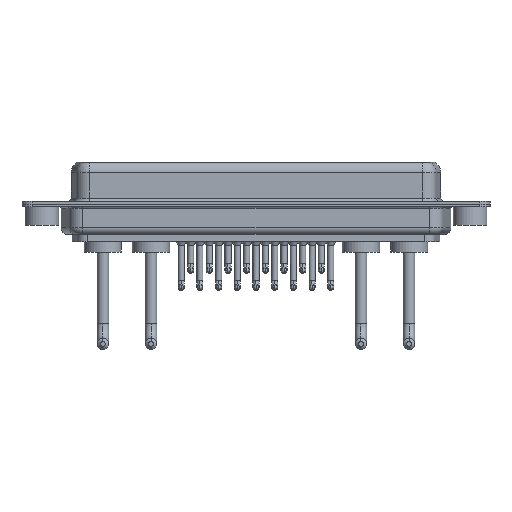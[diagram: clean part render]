
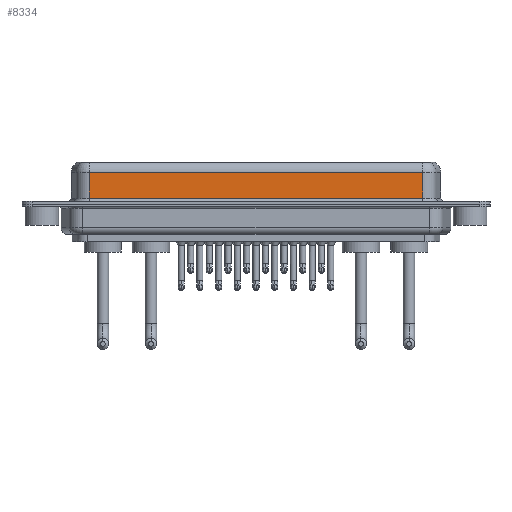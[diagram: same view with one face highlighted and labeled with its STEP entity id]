
A CAD part, front view. The second image highlights one B-rep face of the part: STEP entity #8334.
In plain terms, the highlighted planar face has unit normal (0, -1, 0).
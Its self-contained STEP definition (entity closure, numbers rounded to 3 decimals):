
#662 = ORIENTED_EDGE ( 'NONE', *, *, #8772, .T. ) ;
#1436 = DIRECTION ( 'NONE',  ( -1., 0., 0. ) ) ;
#1782 = DIRECTION ( 'NONE',  ( 0., 0., -1. ) ) ;
#2247 = ORIENTED_EDGE ( 'NONE', *, *, #20388, .F. ) ;
#2934 = EDGE_CURVE ( 'NONE', #20072, #3541, #20333, .T. ) ;
#3494 = CARTESIAN_POINT ( 'NONE',  ( 56.462, -3.95, 0.9 ) ) ;
#3541 = VERTEX_POINT ( 'NONE', #10389 ) ;
#3638 = ORIENTED_EDGE ( 'NONE', *, *, #15720, .T. ) ;
#3712 = PLANE ( 'NONE',  #6332 ) ;
#4052 = ORIENTED_EDGE ( 'NONE', *, *, #2934, .T. ) ;
#4742 = DIRECTION ( 'NONE',  ( 0., 0., 1. ) ) ;
#4967 = VERTEX_POINT ( 'NONE', #16690 ) ;
#5151 = LINE ( 'NONE', #8379, #12789 ) ;
#6005 = VECTOR ( 'NONE', #20217, 1000. ) ;
#6332 = AXIS2_PLACEMENT_3D ( 'NONE', #13130, #20021, #4742 ) ;
#6909 = CARTESIAN_POINT ( 'NONE',  ( 56.462, -3.95, 4.65 ) ) ;
#7437 = CARTESIAN_POINT ( 'NONE',  ( 7.038, -3.95, 4.65 ) ) ;
#7652 = CARTESIAN_POINT ( 'NONE',  ( 7.038, -3.95, 0.9 ) ) ;
#8334 = ADVANCED_FACE ( 'NONE', ( #14922 ), #3712, .F. ) ;
#8379 = CARTESIAN_POINT ( 'NONE',  ( 7.038, -3.95, 6.4 ) ) ;
#8772 = EDGE_CURVE ( 'NONE', #20502, #20072, #5151, .T. ) ;
#10389 = CARTESIAN_POINT ( 'NONE',  ( 56.462, -3.95, 0.9 ) ) ;
#11086 = CARTESIAN_POINT ( 'NONE',  ( 56.462, -3.95, 6.4 ) ) ;
#11422 = LINE ( 'NONE', #11086, #16417 ) ;
#12789 = VECTOR ( 'NONE', #1782, 1000. ) ;
#13130 = CARTESIAN_POINT ( 'NONE',  ( 56.462, -3.95, 6.4 ) ) ;
#14556 = DIRECTION ( 'NONE',  ( 0., 0., -1. ) ) ;
#14922 = FACE_OUTER_BOUND ( 'NONE', #15537, .T. ) ;
#15529 = VECTOR ( 'NONE', #1436, 1000. ) ;
#15537 = EDGE_LOOP ( 'NONE', ( #2247, #3638, #662, #4052 ) ) ;
#15720 = EDGE_CURVE ( 'NONE', #4967, #20502, #21735, .T. ) ;
#16417 = VECTOR ( 'NONE', #14556, 1000. ) ;
#16690 = CARTESIAN_POINT ( 'NONE',  ( 56.462, -3.95, 4.65 ) ) ;
#20021 = DIRECTION ( 'NONE',  ( 0., 1., 0. ) ) ;
#20072 = VERTEX_POINT ( 'NONE', #7652 ) ;
#20217 = DIRECTION ( 'NONE',  ( 1., 0., 0. ) ) ;
#20333 = LINE ( 'NONE', #3494, #6005 ) ;
#20388 = EDGE_CURVE ( 'NONE', #4967, #3541, #11422, .T. ) ;
#20502 = VERTEX_POINT ( 'NONE', #7437 ) ;
#21735 = LINE ( 'NONE', #6909, #15529 ) ;
